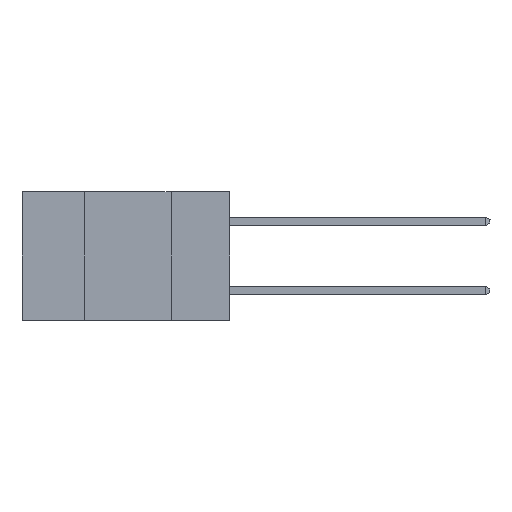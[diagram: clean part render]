
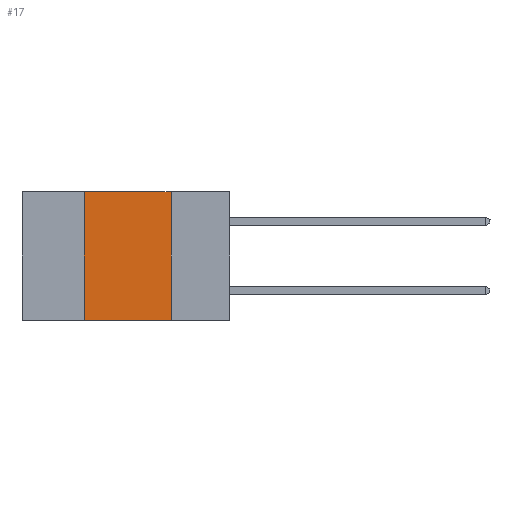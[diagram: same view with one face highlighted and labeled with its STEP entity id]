
A CAD part, left-side view. The second image highlights one B-rep face of the part: STEP entity #17.
In plain terms, the highlighted planar face has unit normal (-1, 0, 0).
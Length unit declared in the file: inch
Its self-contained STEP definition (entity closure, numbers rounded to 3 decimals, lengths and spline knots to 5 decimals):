
#17 = ADVANCED_FACE ( 'NONE', ( #28017 ), #7827, .F. ) ;
#2979 = LINE ( 'NONE', #23109, #26937 ) ;
#3353 = CARTESIAN_POINT ( 'NONE',  ( 0., 0.42, 0. ) ) ;
#3877 = CARTESIAN_POINT ( 'NONE',  ( 0., 0.6, 0. ) ) ;
#3886 = EDGE_CURVE ( 'NONE', #27496, #25949, #10829, .T. ) ;
#6956 = CARTESIAN_POINT ( 'NONE',  ( 0., 0.42, -0.37 ) ) ;
#7311 = EDGE_LOOP ( 'NONE', ( #17018, #29040, #20888, #11843 ) ) ;
#7827 = PLANE ( 'NONE',  #26226 ) ;
#8002 = DIRECTION ( 'NONE',  ( 0., 0., 1. ) ) ;
#10310 = EDGE_CURVE ( 'NONE', #27767, #27496, #2979, .T. ) ;
#10829 = LINE ( 'NONE', #10857, #17378 ) ;
#10857 = CARTESIAN_POINT ( 'NONE',  ( 0., 0.17, 0. ) ) ;
#11843 = ORIENTED_EDGE ( 'NONE', *, *, #17681, .T. ) ;
#12064 = EDGE_CURVE ( 'NONE', #29069, #27767, #15596, .T. ) ;
#15596 = LINE ( 'NONE', #3353, #26454 ) ;
#17018 = ORIENTED_EDGE ( 'NONE', *, *, #3886, .F. ) ;
#17203 = DIRECTION ( 'NONE',  ( 0., -1., 0. ) ) ;
#17378 = VECTOR ( 'NONE', #22611, 39.37008 ) ;
#17544 = CARTESIAN_POINT ( 'NONE',  ( 0., 0.6, -0.37 ) ) ;
#17681 = EDGE_CURVE ( 'NONE', #29069, #25949, #22722, .T. ) ;
#18016 = VECTOR ( 'NONE', #19873, 39.37008 ) ;
#18364 = CARTESIAN_POINT ( 'NONE',  ( 0., 0.17, -0.37 ) ) ;
#19388 = CARTESIAN_POINT ( 'NONE',  ( 0., 0.17, 0. ) ) ;
#19873 = DIRECTION ( 'NONE',  ( 0., -1., 0. ) ) ;
#20888 = ORIENTED_EDGE ( 'NONE', *, *, #12064, .F. ) ;
#22437 = DIRECTION ( 'NONE',  ( 1., 0., 0. ) ) ;
#22611 = DIRECTION ( 'NONE',  ( 0., 0., -1. ) ) ;
#22722 = LINE ( 'NONE', #17544, #18016 ) ;
#22962 = CARTESIAN_POINT ( 'NONE',  ( 0., 0.42, 0. ) ) ;
#23109 = CARTESIAN_POINT ( 'NONE',  ( 0., 0.6, 0. ) ) ;
#24057 = DIRECTION ( 'NONE',  ( 0., 0., -1. ) ) ;
#25949 = VERTEX_POINT ( 'NONE', #18364 ) ;
#26226 = AXIS2_PLACEMENT_3D ( 'NONE', #3877, #22437, #24057 ) ;
#26454 = VECTOR ( 'NONE', #8002, 39.37008 ) ;
#26937 = VECTOR ( 'NONE', #17203, 39.37008 ) ;
#27496 = VERTEX_POINT ( 'NONE', #19388 ) ;
#27767 = VERTEX_POINT ( 'NONE', #22962 ) ;
#28017 = FACE_OUTER_BOUND ( 'NONE', #7311, .T. ) ;
#29040 = ORIENTED_EDGE ( 'NONE', *, *, #10310, .F. ) ;
#29069 = VERTEX_POINT ( 'NONE', #6956 ) ;
